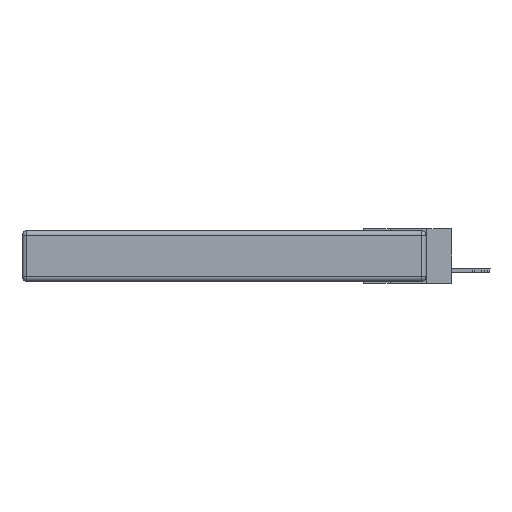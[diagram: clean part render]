
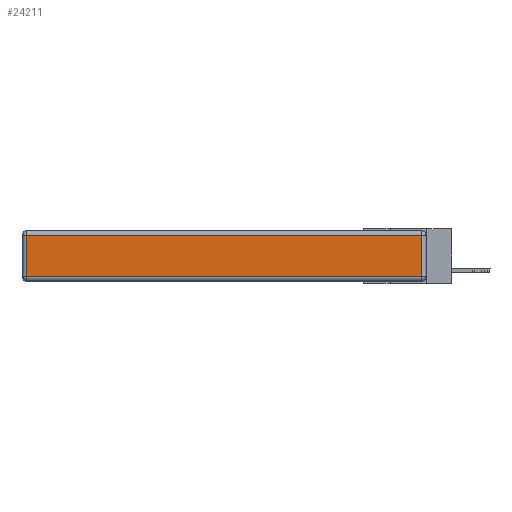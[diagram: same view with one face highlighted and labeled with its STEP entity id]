
A CAD part, left-side view. The second image highlights one B-rep face of the part: STEP entity #24211.
In plain terms, the highlighted planar face has unit normal (-1, 0, 0).
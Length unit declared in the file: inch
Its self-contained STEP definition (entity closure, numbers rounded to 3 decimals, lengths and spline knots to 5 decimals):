
#245 = CARTESIAN_POINT ( 'NONE',  ( 0., 2.72, -0.343 ) ) ;
#525 = LINE ( 'NONE', #8404, #25969 ) ;
#769 = AXIS2_PLACEMENT_3D ( 'NONE', #6692, #14539, #24662 ) ;
#1005 = LINE ( 'NONE', #6255, #10590 ) ;
#1883 = CARTESIAN_POINT ( 'NONE',  ( 0., 2.72, -0.03 ) ) ;
#3101 = VECTOR ( 'NONE', #28943, 39.37008 ) ;
#3412 = DIRECTION ( 'NONE',  ( 0., -1., 0. ) ) ;
#3498 = DIRECTION ( 'NONE',  ( 0., 1., 0. ) ) ;
#4674 = VERTEX_POINT ( 'NONE', #9734 ) ;
#6255 = CARTESIAN_POINT ( 'NONE',  ( 0., 0., -0.313 ) ) ;
#6340 = CARTESIAN_POINT ( 'NONE',  ( 0., 0.03, -0.03 ) ) ;
#6634 = VERTEX_POINT ( 'NONE', #6340 ) ;
#6687 = VERTEX_POINT ( 'NONE', #12755 ) ;
#6692 = CARTESIAN_POINT ( 'NONE',  ( 0., 0., -0.343 ) ) ;
#7106 = LINE ( 'NONE', #10000, #15586 ) ;
#7417 = EDGE_CURVE ( 'NONE', #31112, #6687, #31341, .T. ) ;
#8404 = CARTESIAN_POINT ( 'NONE',  ( 0., 2.75, -0.03 ) ) ;
#9636 = ORIENTED_EDGE ( 'NONE', *, *, #7417, .T. ) ;
#9734 = CARTESIAN_POINT ( 'NONE',  ( 0., 0.03, -0.313 ) ) ;
#10000 = CARTESIAN_POINT ( 'NONE',  ( 0., 0.03, -0.343 ) ) ;
#10590 = VECTOR ( 'NONE', #3412, 39.37008 ) ;
#12755 = CARTESIAN_POINT ( 'NONE',  ( 0., 2.72, -0.313 ) ) ;
#14429 = PLANE ( 'NONE',  #769 ) ;
#14539 = DIRECTION ( 'NONE',  ( -1., 0., 0. ) ) ;
#15165 = DIRECTION ( 'NONE',  ( 0., 0., 1. ) ) ;
#15586 = VECTOR ( 'NONE', #15165, 39.37008 ) ;
#21250 = EDGE_CURVE ( 'NONE', #6634, #31112, #525, .T. ) ;
#23949 = EDGE_LOOP ( 'NONE', ( #32604, #28565, #25922, #9636 ) ) ;
#24211 = ADVANCED_FACE ( 'NONE', ( #32016 ), #14429, .T. ) ;
#24662 = DIRECTION ( 'NONE',  ( 0., 0., 1. ) ) ;
#25922 = ORIENTED_EDGE ( 'NONE', *, *, #21250, .T. ) ;
#25969 = VECTOR ( 'NONE', #3498, 39.37008 ) ;
#28565 = ORIENTED_EDGE ( 'NONE', *, *, #33171, .T. ) ;
#28943 = DIRECTION ( 'NONE',  ( 0., 0., -1. ) ) ;
#29412 = EDGE_CURVE ( 'NONE', #6687, #4674, #1005, .T. ) ;
#31112 = VERTEX_POINT ( 'NONE', #1883 ) ;
#31341 = LINE ( 'NONE', #245, #3101 ) ;
#32016 = FACE_OUTER_BOUND ( 'NONE', #23949, .T. ) ;
#32604 = ORIENTED_EDGE ( 'NONE', *, *, #29412, .T. ) ;
#33171 = EDGE_CURVE ( 'NONE', #4674, #6634, #7106, .T. ) ;
